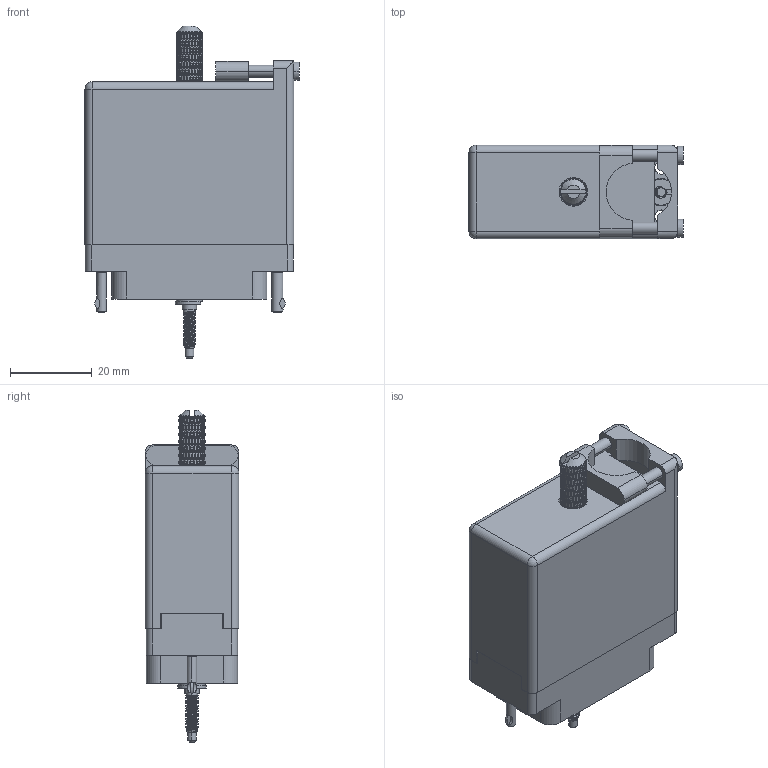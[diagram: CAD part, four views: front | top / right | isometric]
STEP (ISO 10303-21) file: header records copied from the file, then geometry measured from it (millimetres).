
FILE_DESCRIPTION (( 'STEP AP203' ), '1' );
FILE_NAME ('516-038-520-161.STEP', '2020-03-09T21:18:19', ( '' ), ( '' ), 'SwSTEP 2.0', 'SolidWorks 2016', '' );
FILE_SCHEMA (( 'CONFIG_CONTROL_DESIGN' ));
Length unit declared in the file: inch
Products named in the file (12): 516-253-035-100; 516-222-038-102_039; 516-230-001_Metal - 038 Top Entry; 516-222-038-102_038; 516-252-021-102_038; 516-038-520-161; 516-251-035-100; 516 Plug Insulator_038; 516-253-138-107; Actuating Screw Assy 038-056; 516-292-001_520 Contact; 516-250-038-111
Assembly tree (50 placements, depth 3):
  516-038-520-161
    516 Plug Insulator_038
    516-292-001_520 Contact  x38
    516-230-001_Metal - 038 Top Entry
    516-252-021-102_038  x2
    516-222-038-102_038
    Actuating Screw Assy 038-056
      516-251-035-100
      516-253-035-100  x2
      516-253-138-107
      516-250-038-111
    516-222-038-102_039
Bounding box: 52.27 x 22.83 x 81.03 mm (x, y, z)
Volume: 21499.1 mm3; surface area: 34615 mm2
Topology: 49 solids, 49 shells, 5269 faces, 14146 edges, 8996 vertices
Faces by surface type: plane 2390, cylinder 1549, bspline 1270, cone 54, torus 4, sphere 2
Entity records: 111701 total; most frequent: CARTESIAN_POINT 60081, ORIENTED_EDGE 12692, DIRECTION 7663, EDGE_CURVE 6346, VERTEX_POINT 3822, EDGE_LOOP 2700, AXIS2_PLACEMENT_3D 2622, FACE_OUTER_BOUND 2568
